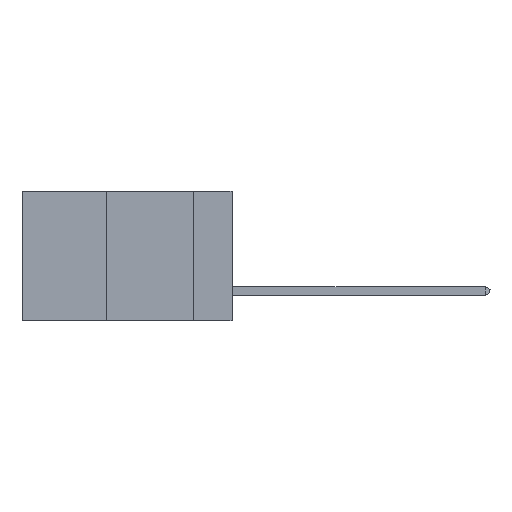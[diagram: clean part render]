
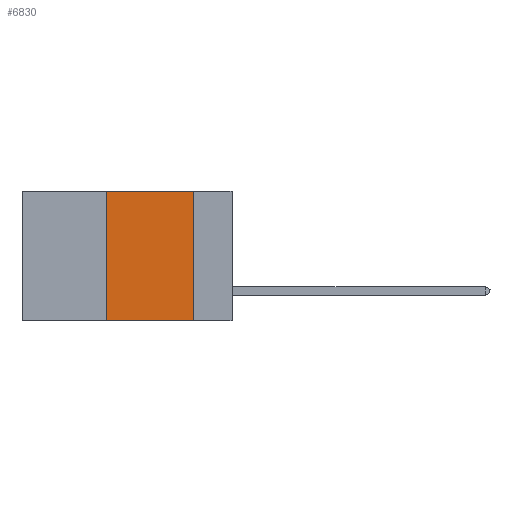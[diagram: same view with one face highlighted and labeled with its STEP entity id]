
A CAD part, left-side view. The second image highlights one B-rep face of the part: STEP entity #6830.
In plain terms, the highlighted planar face has unit normal (-1, 0, 0).
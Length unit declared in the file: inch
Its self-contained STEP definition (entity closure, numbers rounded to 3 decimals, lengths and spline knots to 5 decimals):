
#200 = CARTESIAN_POINT ( 'NONE',  ( 0., 0.11, 0. ) ) ;
#211 = LINE ( 'NONE', #19415, #9928 ) ;
#269 = LINE ( 'NONE', #12139, #6124 ) ;
#1850 = CARTESIAN_POINT ( 'NONE',  ( 0., 0.11, 0. ) ) ;
#2473 = ORIENTED_EDGE ( 'NONE', *, *, #18442, .F. ) ;
#2898 = CARTESIAN_POINT ( 'NONE',  ( 0., 0.11, -0.37 ) ) ;
#2902 = DIRECTION ( 'NONE',  ( 0., 0., -1. ) ) ;
#3131 = PLANE ( 'NONE',  #21719 ) ;
#3133 = ORIENTED_EDGE ( 'NONE', *, *, #13688, .T. ) ;
#3294 = ORIENTED_EDGE ( 'NONE', *, *, #17105, .F. ) ;
#4792 = LINE ( 'NONE', #19661, #20832 ) ;
#5050 = EDGE_LOOP ( 'NONE', ( #5653, #2473, #3294, #3133 ) ) ;
#5239 = VERTEX_POINT ( 'NONE', #2898 ) ;
#5262 = DIRECTION ( 'NONE',  ( 0., 0., -1. ) ) ;
#5412 = DIRECTION ( 'NONE',  ( 0., -1., 0. ) ) ;
#5653 = ORIENTED_EDGE ( 'NONE', *, *, #6305, .F. ) ;
#5742 = LINE ( 'NONE', #200, #7669 ) ;
#6124 = VECTOR ( 'NONE', #6729, 39.37008 ) ;
#6305 = EDGE_CURVE ( 'NONE', #10870, #5239, #5742, .T. ) ;
#6604 = CARTESIAN_POINT ( 'NONE',  ( 0., 0.36, 0. ) ) ;
#6729 = DIRECTION ( 'NONE',  ( 0., 0., 1. ) ) ;
#6830 = ADVANCED_FACE ( 'NONE', ( #14834 ), #3131, .F. ) ;
#7669 = VECTOR ( 'NONE', #5262, 39.37008 ) ;
#9046 = VERTEX_POINT ( 'NONE', #14913 ) ;
#9928 = VECTOR ( 'NONE', #5412, 39.37008 ) ;
#10115 = DIRECTION ( 'NONE',  ( 1., 0., 0. ) ) ;
#10870 = VERTEX_POINT ( 'NONE', #1850 ) ;
#12139 = CARTESIAN_POINT ( 'NONE',  ( 0., 0.36, 0. ) ) ;
#13079 = VERTEX_POINT ( 'NONE', #6604 ) ;
#13688 = EDGE_CURVE ( 'NONE', #9046, #5239, #4792, .T. ) ;
#14834 = FACE_OUTER_BOUND ( 'NONE', #5050, .T. ) ;
#14913 = CARTESIAN_POINT ( 'NONE',  ( 0., 0.36, -0.37 ) ) ;
#15343 = CARTESIAN_POINT ( 'NONE',  ( 0., 0.6, 0. ) ) ;
#17105 = EDGE_CURVE ( 'NONE', #9046, #13079, #269, .T. ) ;
#17866 = DIRECTION ( 'NONE',  ( 0., -1., 0. ) ) ;
#18442 = EDGE_CURVE ( 'NONE', #13079, #10870, #211, .T. ) ;
#19415 = CARTESIAN_POINT ( 'NONE',  ( 0., 0.6, 0. ) ) ;
#19661 = CARTESIAN_POINT ( 'NONE',  ( 0., 0.6, -0.37 ) ) ;
#20832 = VECTOR ( 'NONE', #17866, 39.37008 ) ;
#21719 = AXIS2_PLACEMENT_3D ( 'NONE', #15343, #10115, #2902 ) ;
